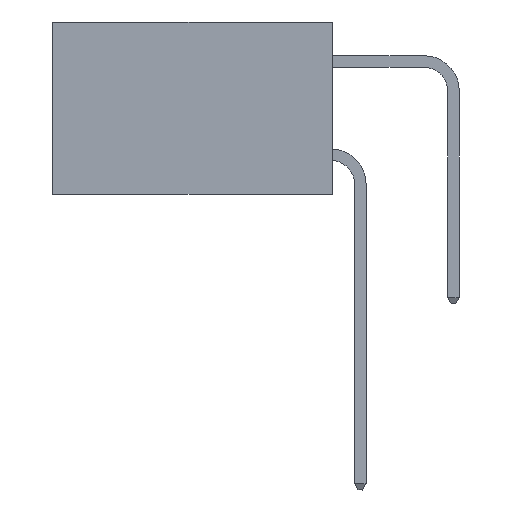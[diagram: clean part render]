
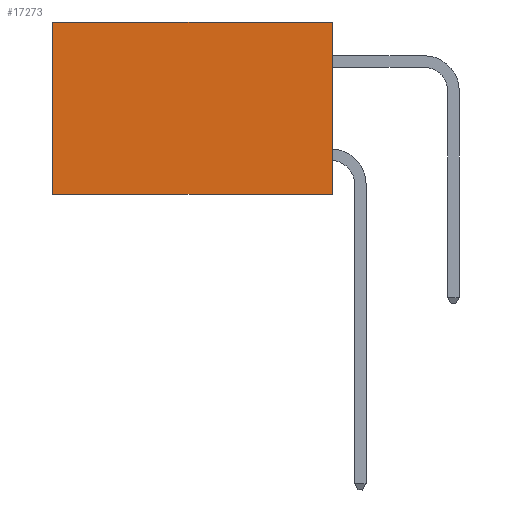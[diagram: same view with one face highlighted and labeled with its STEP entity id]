
A CAD part, left-side view. The second image highlights one B-rep face of the part: STEP entity #17273.
In plain terms, the highlighted planar face has unit normal (-1, 0, 0).
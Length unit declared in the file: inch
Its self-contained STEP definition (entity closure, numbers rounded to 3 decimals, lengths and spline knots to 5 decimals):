
#270 = EDGE_CURVE ( 'NONE', #10911, #13545, #13555, .T. ) ;
#798 = VECTOR ( 'NONE', #20489, 39.37008 ) ;
#1505 = VECTOR ( 'NONE', #16199, 39.37008 ) ;
#2757 = EDGE_LOOP ( 'NONE', ( #6158, #17186, #2997, #4744 ) ) ;
#2851 = EDGE_CURVE ( 'NONE', #15838, #10911, #9318, .T. ) ;
#2997 = ORIENTED_EDGE ( 'NONE', *, *, #2851, .F. ) ;
#4744 = ORIENTED_EDGE ( 'NONE', *, *, #18500, .T. ) ;
#5017 = FACE_OUTER_BOUND ( 'NONE', #2757, .T. ) ;
#6158 = ORIENTED_EDGE ( 'NONE', *, *, #19656, .T. ) ;
#7926 = VERTEX_POINT ( 'NONE', #9944 ) ;
#9318 = LINE ( 'NONE', #14194, #21044 ) ;
#9933 = CARTESIAN_POINT ( 'NONE',  ( 0.2615, 0., -0.37 ) ) ;
#9944 = CARTESIAN_POINT ( 'NONE',  ( 0.2615, 0.6, 0. ) ) ;
#9976 = AXIS2_PLACEMENT_3D ( 'NONE', #13517, #21515, #20113 ) ;
#10911 = VERTEX_POINT ( 'NONE', #20550 ) ;
#13249 = LINE ( 'NONE', #18585, #16108 ) ;
#13517 = CARTESIAN_POINT ( 'NONE',  ( 0.2615, 0., -0.37 ) ) ;
#13545 = VERTEX_POINT ( 'NONE', #18466 ) ;
#13555 = LINE ( 'NONE', #9933, #798 ) ;
#13577 = DIRECTION ( 'NONE',  ( 0., 0., -1. ) ) ;
#14149 = CARTESIAN_POINT ( 'NONE',  ( 0.2615, 0., 0. ) ) ;
#14194 = CARTESIAN_POINT ( 'NONE',  ( 0.2615, 0., -0.37 ) ) ;
#15119 = CARTESIAN_POINT ( 'NONE',  ( 0.2615, 0., 0. ) ) ;
#15838 = VERTEX_POINT ( 'NONE', #15119 ) ;
#16108 = VECTOR ( 'NONE', #13577, 39.37008 ) ;
#16131 = DIRECTION ( 'NONE',  ( 0., 0., -1. ) ) ;
#16199 = DIRECTION ( 'NONE',  ( 0., 1., 0. ) ) ;
#17053 = PLANE ( 'NONE',  #9976 ) ;
#17186 = ORIENTED_EDGE ( 'NONE', *, *, #270, .F. ) ;
#17273 = ADVANCED_FACE ( 'NONE', ( #5017 ), #17053, .F. ) ;
#18466 = CARTESIAN_POINT ( 'NONE',  ( 0.2615, 0.6, -0.37 ) ) ;
#18500 = EDGE_CURVE ( 'NONE', #15838, #7926, #21310, .T. ) ;
#18585 = CARTESIAN_POINT ( 'NONE',  ( 0.2615, 0.6, -0.37 ) ) ;
#19656 = EDGE_CURVE ( 'NONE', #7926, #13545, #13249, .T. ) ;
#20113 = DIRECTION ( 'NONE',  ( 0., 0., -1. ) ) ;
#20489 = DIRECTION ( 'NONE',  ( 0., 1., 0. ) ) ;
#20550 = CARTESIAN_POINT ( 'NONE',  ( 0.2615, 0., -0.37 ) ) ;
#21044 = VECTOR ( 'NONE', #16131, 39.37008 ) ;
#21310 = LINE ( 'NONE', #14149, #1505 ) ;
#21515 = DIRECTION ( 'NONE',  ( 1., 0., 0. ) ) ;
